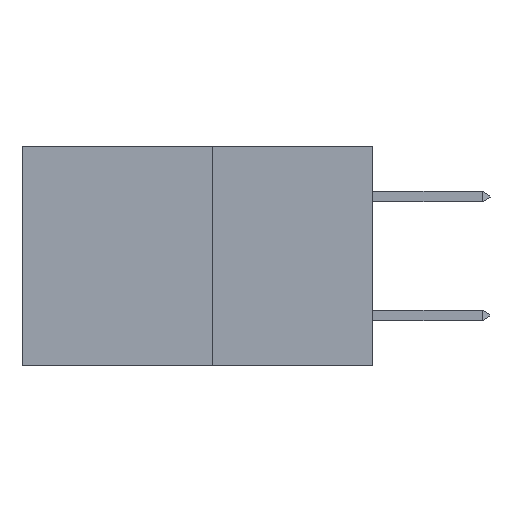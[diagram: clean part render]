
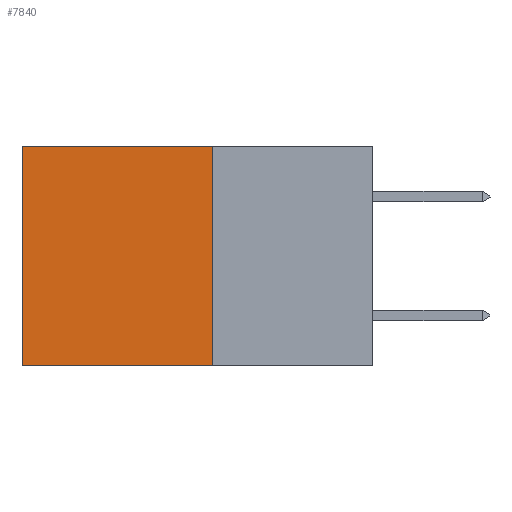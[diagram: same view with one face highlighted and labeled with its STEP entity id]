
A CAD part, left-side view. The second image highlights one B-rep face of the part: STEP entity #7840.
In plain terms, the highlighted planar face has unit normal (-1, 0, 0).
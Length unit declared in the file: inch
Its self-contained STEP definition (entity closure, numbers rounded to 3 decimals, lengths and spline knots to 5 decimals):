
#177 = ORIENTED_EDGE ( 'NONE', *, *, #12671, .T. ) ;
#309 = EDGE_CURVE ( 'NONE', #2900, #6497, #6040, .T. ) ;
#881 = CARTESIAN_POINT ( 'NONE',  ( 0.277, 0.27, -0.37 ) ) ;
#1413 = LINE ( 'NONE', #2721, #10771 ) ;
#1420 = CARTESIAN_POINT ( 'NONE',  ( 0.277, 0.27, 0. ) ) ;
#2291 = AXIS2_PLACEMENT_3D ( 'NONE', #4159, #3787, #3953 ) ;
#2409 = DIRECTION ( 'NONE',  ( 0., 0., -1. ) ) ;
#2594 = CARTESIAN_POINT ( 'NONE',  ( 0.277, 0.59, 0. ) ) ;
#2721 = CARTESIAN_POINT ( 'NONE',  ( 0.277, 0.59, -0.37 ) ) ;
#2873 = LINE ( 'NONE', #14627, #15098 ) ;
#2900 = VERTEX_POINT ( 'NONE', #1420 ) ;
#3141 = CARTESIAN_POINT ( 'NONE',  ( 0.277, 0.59, -0.37 ) ) ;
#3280 = DIRECTION ( 'NONE',  ( 0., 1., 0. ) ) ;
#3766 = EDGE_CURVE ( 'NONE', #15643, #8728, #14205, .T. ) ;
#3787 = DIRECTION ( 'NONE',  ( 1., 0., 0. ) ) ;
#3953 = DIRECTION ( 'NONE',  ( 0., 0., -1. ) ) ;
#4159 = CARTESIAN_POINT ( 'NONE',  ( 0.277, 0.27, -0.37 ) ) ;
#6039 = EDGE_LOOP ( 'NONE', ( #177, #10347, #8476, #7395 ) ) ;
#6040 = LINE ( 'NONE', #8614, #13892 ) ;
#6497 = VERTEX_POINT ( 'NONE', #2594 ) ;
#7395 = ORIENTED_EDGE ( 'NONE', *, *, #309, .T. ) ;
#7821 = DIRECTION ( 'NONE',  ( 0., 1., 0. ) ) ;
#7840 = ADVANCED_FACE ( 'NONE', ( #12060 ), #11194, .F. ) ;
#8476 = ORIENTED_EDGE ( 'NONE', *, *, #13040, .F. ) ;
#8614 = CARTESIAN_POINT ( 'NONE',  ( 0.277, 0.27, 0. ) ) ;
#8728 = VERTEX_POINT ( 'NONE', #3141 ) ;
#10347 = ORIENTED_EDGE ( 'NONE', *, *, #3766, .F. ) ;
#10771 = VECTOR ( 'NONE', #2409, 39.37008 ) ;
#11194 = PLANE ( 'NONE',  #2291 ) ;
#12060 = FACE_OUTER_BOUND ( 'NONE', #6039, .T. ) ;
#12356 = CARTESIAN_POINT ( 'NONE',  ( 0.277, 0.27, -0.37 ) ) ;
#12671 = EDGE_CURVE ( 'NONE', #6497, #8728, #1413, .T. ) ;
#13040 = EDGE_CURVE ( 'NONE', #2900, #15643, #2873, .T. ) ;
#13823 = VECTOR ( 'NONE', #7821, 39.37008 ) ;
#13892 = VECTOR ( 'NONE', #3280, 39.37008 ) ;
#14205 = LINE ( 'NONE', #881, #13823 ) ;
#14577 = DIRECTION ( 'NONE',  ( 0., 0., -1. ) ) ;
#14627 = CARTESIAN_POINT ( 'NONE',  ( 0.277, 0.27, -0.37 ) ) ;
#15098 = VECTOR ( 'NONE', #14577, 39.37008 ) ;
#15643 = VERTEX_POINT ( 'NONE', #12356 ) ;
